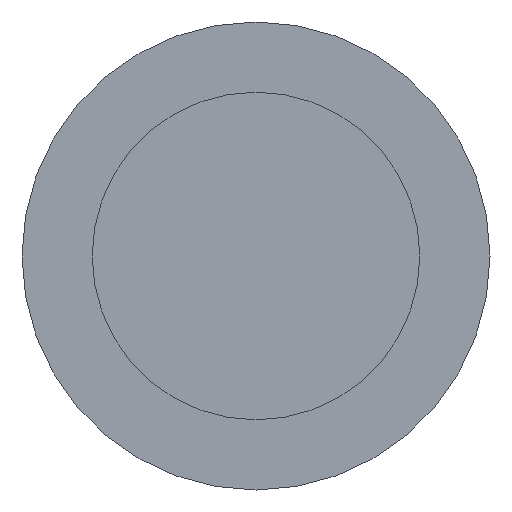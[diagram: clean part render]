
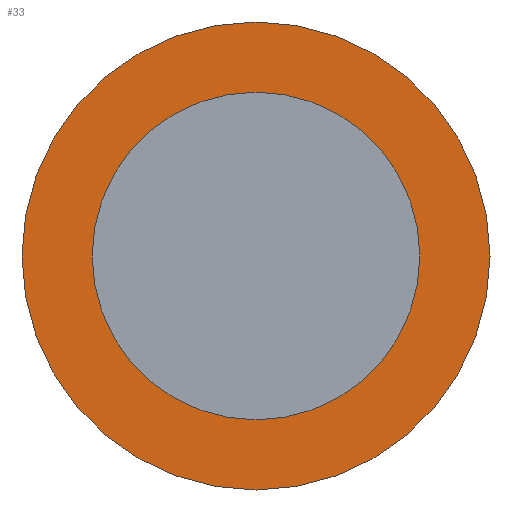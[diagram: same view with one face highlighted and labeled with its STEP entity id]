
A CAD part, front view. The second image highlights one B-rep face of the part: STEP entity #33.
In plain terms, the highlighted planar face has unit normal (0, -1, 0).
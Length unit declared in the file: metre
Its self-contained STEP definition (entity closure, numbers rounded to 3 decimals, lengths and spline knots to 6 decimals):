
#33 = ADVANCED_FACE( '', ( #62, #63 ), #64, .T. );
#62 = FACE_OUTER_BOUND( '', #87, .T. );
#63 = FACE_BOUND( '', #88, .T. );
#64 = PLANE( '', #89 );
#87 = EDGE_LOOP( '', ( #110 ) );
#88 = EDGE_LOOP( '', ( #111 ) );
#89 = AXIS2_PLACEMENT_3D( '', #112, #113, #114 );
#110 = ORIENTED_EDGE( '', *, *, #132, .T. );
#111 = ORIENTED_EDGE( '', *, *, #133, .F. );
#112 = CARTESIAN_POINT( '', ( 0.003175, -0.00254, 0. ) );
#113 = DIRECTION( '', ( 0., -1., 0. ) );
#114 = DIRECTION( '', ( 0., 0., -1. ) );
#132 = EDGE_CURVE( '', #143, #143, #144, .T. );
#133 = EDGE_CURVE( '', #145, #145, #146, .T. );
#143 = VERTEX_POINT( '', #156 );
#144 = CIRCLE( '', #157, 0.003175 );
#145 = VERTEX_POINT( '', #158 );
#146 = CIRCLE( '', #159, 0.002223 );
#156 = CARTESIAN_POINT( '', ( 0., -0.00254, -0.003175 ) );
#157 = AXIS2_PLACEMENT_3D( '', #168, #169, #170 );
#158 = CARTESIAN_POINT( '', ( 0., -0.00254, -0.002223 ) );
#159 = AXIS2_PLACEMENT_3D( '', #171, #172, #173 );
#168 = CARTESIAN_POINT( '', ( 0., -0.00254, 0. ) );
#169 = DIRECTION( '', ( 0., -1., 0. ) );
#170 = DIRECTION( '', ( 0., 0., -1. ) );
#171 = CARTESIAN_POINT( '', ( 0., -0.00254, 0. ) );
#172 = DIRECTION( '', ( 0., -1., 0. ) );
#173 = DIRECTION( '', ( 0., 0., -1. ) );
